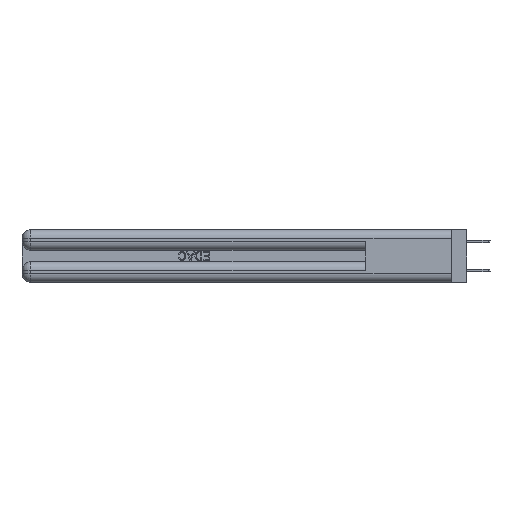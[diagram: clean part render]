
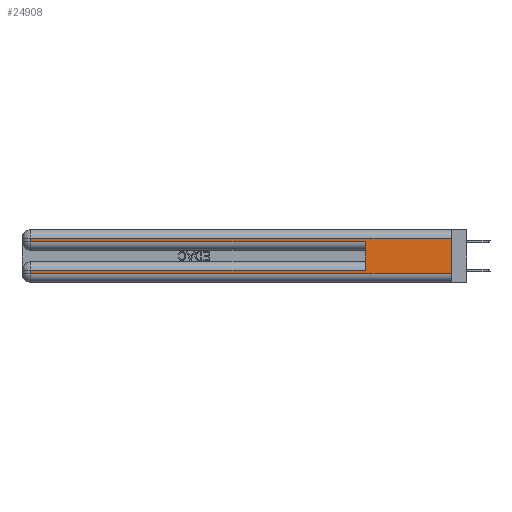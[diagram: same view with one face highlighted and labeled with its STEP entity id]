
A CAD part, left-side view. The second image highlights one B-rep face of the part: STEP entity #24908.
In plain terms, the highlighted planar face has unit normal (-1, 0, 0).
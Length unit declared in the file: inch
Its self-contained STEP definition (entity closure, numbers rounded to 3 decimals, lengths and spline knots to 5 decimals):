
#2545 = CARTESIAN_POINT ( 'NONE',  ( 0., 0., 0.31 ) ) ;
#2879 = VERTEX_POINT ( 'NONE', #34968 ) ;
#5394 = CARTESIAN_POINT ( 'NONE',  ( 0., 2.94, 0.37 ) ) ;
#6032 = DIRECTION ( 'NONE',  ( 0., 1., 0. ) ) ;
#6405 = CARTESIAN_POINT ( 'NONE',  ( 0., 2.94, 0.31 ) ) ;
#6764 = EDGE_CURVE ( 'NONE', #20034, #16547, #24182, .T. ) ;
#7769 = VECTOR ( 'NONE', #18780, 39.37008 ) ;
#7854 = ORIENTED_EDGE ( 'NONE', *, *, #17851, .T. ) ;
#8087 = ORIENTED_EDGE ( 'NONE', *, *, #19339, .T. ) ;
#9141 = VERTEX_POINT ( 'NONE', #28332 ) ;
#9433 = EDGE_CURVE ( 'NONE', #38739, #23347, #29092, .T. ) ;
#9719 = CARTESIAN_POINT ( 'NONE',  ( 0., 2.94, 0.37 ) ) ;
#10226 = VECTOR ( 'NONE', #36123, 39.37008 ) ;
#10988 = CARTESIAN_POINT ( 'NONE',  ( 0., 0., 0.06 ) ) ;
#11672 = VECTOR ( 'NONE', #35578, 39.37008 ) ;
#11978 = ORIENTED_EDGE ( 'NONE', *, *, #19584, .F. ) ;
#13314 = VERTEX_POINT ( 'NONE', #38883 ) ;
#13453 = EDGE_CURVE ( 'NONE', #23390, #9141, #29859, .T. ) ;
#14874 = DIRECTION ( 'NONE',  ( 0., 0., -1. ) ) ;
#14949 = CARTESIAN_POINT ( 'NONE',  ( 0., 0., 0.285 ) ) ;
#16385 = DIRECTION ( 'NONE',  ( 0., 0., -1. ) ) ;
#16547 = VERTEX_POINT ( 'NONE', #10988 ) ;
#17389 = CARTESIAN_POINT ( 'NONE',  ( 0., 2.94, 0.06 ) ) ;
#17583 = VECTOR ( 'NONE', #33148, 39.37008 ) ;
#17851 = EDGE_CURVE ( 'NONE', #13314, #38739, #27579, .T. ) ;
#18780 = DIRECTION ( 'NONE',  ( 0., -1., 0. ) ) ;
#18810 = CARTESIAN_POINT ( 'NONE',  ( 0., 2.94, 0.285 ) ) ;
#18864 = DIRECTION ( 'NONE',  ( 0., 1., 0. ) ) ;
#19339 = EDGE_CURVE ( 'NONE', #9141, #20034, #33944, .T. ) ;
#19584 = EDGE_CURVE ( 'NONE', #13314, #16547, #21928, .T. ) ;
#19813 = VECTOR ( 'NONE', #14874, 39.37008 ) ;
#20034 = VERTEX_POINT ( 'NONE', #17389 ) ;
#20575 = VECTOR ( 'NONE', #18864, 39.37008 ) ;
#21928 = LINE ( 'NONE', #42571, #23061 ) ;
#23061 = VECTOR ( 'NONE', #36069, 39.37008 ) ;
#23347 = VERTEX_POINT ( 'NONE', #18810 ) ;
#23390 = VERTEX_POINT ( 'NONE', #26122 ) ;
#24182 = LINE ( 'NONE', #28924, #11672 ) ;
#24908 = ADVANCED_FACE ( 'NONE', ( #26185 ), #43731, .F. ) ;
#25699 = ORIENTED_EDGE ( 'NONE', *, *, #13453, .T. ) ;
#26122 = CARTESIAN_POINT ( 'NONE',  ( 0., 0.6, 0.085 ) ) ;
#26185 = FACE_OUTER_BOUND ( 'NONE', #35020, .T. ) ;
#26835 = EDGE_CURVE ( 'NONE', #23390, #2879, #34660, .T. ) ;
#27156 = ORIENTED_EDGE ( 'NONE', *, *, #44134, .T. ) ;
#27579 = LINE ( 'NONE', #2545, #40582 ) ;
#28332 = CARTESIAN_POINT ( 'NONE',  ( 0., 2.94, 0.085 ) ) ;
#28741 = ORIENTED_EDGE ( 'NONE', *, *, #9433, .T. ) ;
#28924 = CARTESIAN_POINT ( 'NONE',  ( 0., 0., 0.06 ) ) ;
#29092 = LINE ( 'NONE', #9719, #19813 ) ;
#29566 = ORIENTED_EDGE ( 'NONE', *, *, #26835, .F. ) ;
#29859 = LINE ( 'NONE', #39504, #20575 ) ;
#33148 = DIRECTION ( 'NONE',  ( 0., 0., -1. ) ) ;
#33432 = CARTESIAN_POINT ( 'NONE',  ( 0., 0., 0.37 ) ) ;
#33944 = LINE ( 'NONE', #5394, #17583 ) ;
#34660 = LINE ( 'NONE', #39741, #10226 ) ;
#34968 = CARTESIAN_POINT ( 'NONE',  ( 0., 0.6, 0.285 ) ) ;
#35020 = EDGE_LOOP ( 'NONE', ( #11978, #7854, #28741, #27156, #29566, #25699, #8087, #43926 ) ) ;
#35578 = DIRECTION ( 'NONE',  ( 0., -1., 0. ) ) ;
#36069 = DIRECTION ( 'NONE',  ( 0., 0., -1. ) ) ;
#36123 = DIRECTION ( 'NONE',  ( 0., 0., 1. ) ) ;
#38739 = VERTEX_POINT ( 'NONE', #6405 ) ;
#38883 = CARTESIAN_POINT ( 'NONE',  ( 0., 0., 0.31 ) ) ;
#39243 = LINE ( 'NONE', #14949, #7769 ) ;
#39504 = CARTESIAN_POINT ( 'NONE',  ( 0., 0., 0.085 ) ) ;
#39741 = CARTESIAN_POINT ( 'NONE',  ( 0., 0.6, 0.145 ) ) ;
#40582 = VECTOR ( 'NONE', #6032, 39.37008 ) ;
#41985 = AXIS2_PLACEMENT_3D ( 'NONE', #33432, #43879, #16385 ) ;
#42571 = CARTESIAN_POINT ( 'NONE',  ( 0., 0., 0.37 ) ) ;
#43731 = PLANE ( 'NONE',  #41985 ) ;
#43879 = DIRECTION ( 'NONE',  ( 1., 0., 0. ) ) ;
#43926 = ORIENTED_EDGE ( 'NONE', *, *, #6764, .T. ) ;
#44134 = EDGE_CURVE ( 'NONE', #23347, #2879, #39243, .T. ) ;
